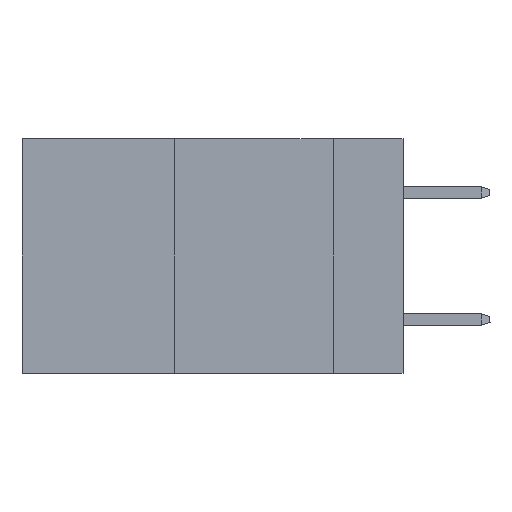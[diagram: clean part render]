
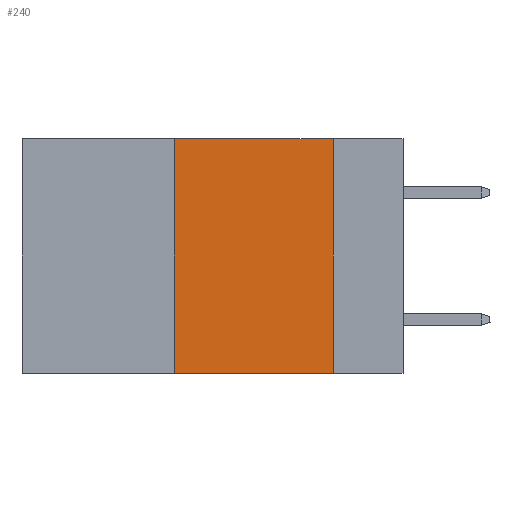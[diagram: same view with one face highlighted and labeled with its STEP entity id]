
A CAD part, left-side view. The second image highlights one B-rep face of the part: STEP entity #240.
In plain terms, the highlighted planar face has unit normal (-1, 0, 0).
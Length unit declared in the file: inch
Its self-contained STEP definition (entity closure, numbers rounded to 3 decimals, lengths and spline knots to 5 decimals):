
#240 = ADVANCED_FACE ( 'NONE', ( #9863 ), #13457, .F. ) ;
#642 = DIRECTION ( 'NONE',  ( 0., 0., -1. ) ) ;
#871 = CARTESIAN_POINT ( 'NONE',  ( 0., 0.11, 0. ) ) ;
#2605 = EDGE_CURVE ( 'NONE', #9070, #20669, #6084, .T. ) ;
#3787 = LINE ( 'NONE', #6925, #19900 ) ;
#4212 = CARTESIAN_POINT ( 'NONE',  ( 0., 0.6, 0. ) ) ;
#5191 = CARTESIAN_POINT ( 'NONE',  ( 0., 0.11, -0.37 ) ) ;
#5843 = ORIENTED_EDGE ( 'NONE', *, *, #9157, .F. ) ;
#6084 = LINE ( 'NONE', #19911, #22640 ) ;
#6370 = LINE ( 'NONE', #8536, #8148 ) ;
#6566 = VECTOR ( 'NONE', #642, 39.37008 ) ;
#6925 = CARTESIAN_POINT ( 'NONE',  ( 0., 0.6, -0.37 ) ) ;
#7260 = DIRECTION ( 'NONE',  ( 0., -1., 0. ) ) ;
#8148 = VECTOR ( 'NONE', #15449, 39.37008 ) ;
#8536 = CARTESIAN_POINT ( 'NONE',  ( 0., 0.6, 0. ) ) ;
#9070 = VERTEX_POINT ( 'NONE', #16403 ) ;
#9157 = EDGE_CURVE ( 'NONE', #20669, #9508, #6370, .T. ) ;
#9508 = VERTEX_POINT ( 'NONE', #871 ) ;
#9634 = CARTESIAN_POINT ( 'NONE',  ( 0., 0.11, 0. ) ) ;
#9718 = CARTESIAN_POINT ( 'NONE',  ( 0., 0.36, 0. ) ) ;
#9863 = FACE_OUTER_BOUND ( 'NONE', #13764, .T. ) ;
#10725 = ORIENTED_EDGE ( 'NONE', *, *, #2605, .F. ) ;
#11704 = DIRECTION ( 'NONE',  ( 0., 0., -1. ) ) ;
#12629 = VERTEX_POINT ( 'NONE', #5191 ) ;
#12777 = DIRECTION ( 'NONE',  ( 0., 0., 1. ) ) ;
#13457 = PLANE ( 'NONE',  #17418 ) ;
#13764 = EDGE_LOOP ( 'NONE', ( #14330, #5843, #10725, #21690 ) ) ;
#14330 = ORIENTED_EDGE ( 'NONE', *, *, #15742, .F. ) ;
#15449 = DIRECTION ( 'NONE',  ( 0., -1., 0. ) ) ;
#15742 = EDGE_CURVE ( 'NONE', #9508, #12629, #18416, .T. ) ;
#16403 = CARTESIAN_POINT ( 'NONE',  ( 0., 0.36, -0.37 ) ) ;
#17418 = AXIS2_PLACEMENT_3D ( 'NONE', #4212, #18745, #11704 ) ;
#18416 = LINE ( 'NONE', #9634, #6566 ) ;
#18745 = DIRECTION ( 'NONE',  ( 1., 0., 0. ) ) ;
#19900 = VECTOR ( 'NONE', #7260, 39.37008 ) ;
#19911 = CARTESIAN_POINT ( 'NONE',  ( 0., 0.36, 0. ) ) ;
#20669 = VERTEX_POINT ( 'NONE', #9718 ) ;
#20857 = EDGE_CURVE ( 'NONE', #9070, #12629, #3787, .T. ) ;
#21690 = ORIENTED_EDGE ( 'NONE', *, *, #20857, .T. ) ;
#22640 = VECTOR ( 'NONE', #12777, 39.37008 ) ;
